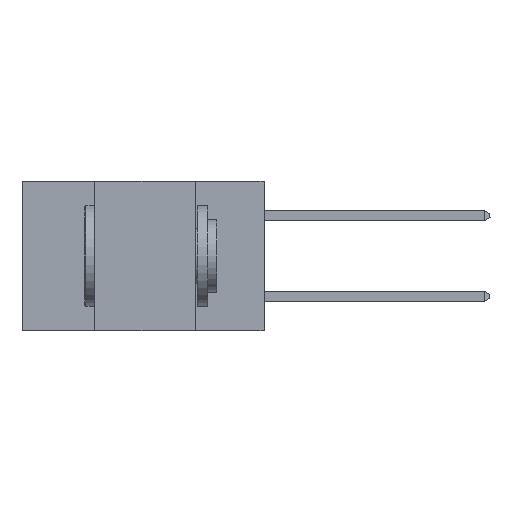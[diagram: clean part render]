
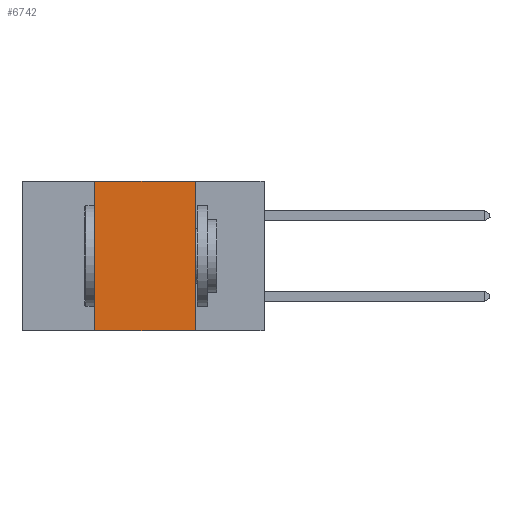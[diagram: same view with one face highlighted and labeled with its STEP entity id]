
A CAD part, left-side view. The second image highlights one B-rep face of the part: STEP entity #6742.
In plain terms, the highlighted planar face has unit normal (-1, 0, 0).
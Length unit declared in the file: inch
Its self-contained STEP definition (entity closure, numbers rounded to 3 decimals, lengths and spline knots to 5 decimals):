
#125 = VERTEX_POINT ( 'NONE', #1342 ) ;
#376 = CARTESIAN_POINT ( 'NONE',  ( 0., 0.42, -0.37 ) ) ;
#1066 = CARTESIAN_POINT ( 'NONE',  ( 0., 0.42, 0. ) ) ;
#1342 = CARTESIAN_POINT ( 'NONE',  ( 0., 0.17, 0. ) ) ;
#1451 = VECTOR ( 'NONE', #9881, 39.37008 ) ;
#2041 = FACE_OUTER_BOUND ( 'NONE', #3314, .T. ) ;
#2465 = AXIS2_PLACEMENT_3D ( 'NONE', #7060, #9429, #7984 ) ;
#2867 = VERTEX_POINT ( 'NONE', #376 ) ;
#2942 = CARTESIAN_POINT ( 'NONE',  ( 0., 0.6, -0.37 ) ) ;
#2954 = CARTESIAN_POINT ( 'NONE',  ( 0., 0.17, 0. ) ) ;
#3314 = EDGE_LOOP ( 'NONE', ( #8979, #4608, #4583, #7929 ) ) ;
#3330 = VERTEX_POINT ( 'NONE', #1066 ) ;
#3410 = VECTOR ( 'NONE', #5240, 39.37008 ) ;
#3616 = LINE ( 'NONE', #4396, #5710 ) ;
#3689 = EDGE_CURVE ( 'NONE', #3330, #125, #6732, .T. ) ;
#3970 = PLANE ( 'NONE',  #2465 ) ;
#4346 = CARTESIAN_POINT ( 'NONE',  ( 0., 0.17, -0.37 ) ) ;
#4396 = CARTESIAN_POINT ( 'NONE',  ( 0., 0.42, 0. ) ) ;
#4583 = ORIENTED_EDGE ( 'NONE', *, *, #6539, .F. ) ;
#4608 = ORIENTED_EDGE ( 'NONE', *, *, #3689, .F. ) ;
#5240 = DIRECTION ( 'NONE',  ( 0., -1., 0. ) ) ;
#5438 = VECTOR ( 'NONE', #8628, 39.37008 ) ;
#5710 = VECTOR ( 'NONE', #9916, 39.37008 ) ;
#5762 = VERTEX_POINT ( 'NONE', #4346 ) ;
#5981 = EDGE_CURVE ( 'NONE', #125, #5762, #9839, .T. ) ;
#6539 = EDGE_CURVE ( 'NONE', #2867, #3330, #3616, .T. ) ;
#6732 = LINE ( 'NONE', #9871, #3410 ) ;
#6742 = ADVANCED_FACE ( 'NONE', ( #2041 ), #3970, .F. ) ;
#7060 = CARTESIAN_POINT ( 'NONE',  ( 0., 0.6, 0. ) ) ;
#7929 = ORIENTED_EDGE ( 'NONE', *, *, #9441, .T. ) ;
#7984 = DIRECTION ( 'NONE',  ( 0., 0., -1. ) ) ;
#8628 = DIRECTION ( 'NONE',  ( 0., 0., -1. ) ) ;
#8979 = ORIENTED_EDGE ( 'NONE', *, *, #5981, .F. ) ;
#9429 = DIRECTION ( 'NONE',  ( 1., 0., 0. ) ) ;
#9441 = EDGE_CURVE ( 'NONE', #2867, #5762, #9658, .T. ) ;
#9658 = LINE ( 'NONE', #2942, #1451 ) ;
#9839 = LINE ( 'NONE', #2954, #5438 ) ;
#9871 = CARTESIAN_POINT ( 'NONE',  ( 0., 0.6, 0. ) ) ;
#9881 = DIRECTION ( 'NONE',  ( 0., -1., 0. ) ) ;
#9916 = DIRECTION ( 'NONE',  ( 0., 0., 1. ) ) ;
